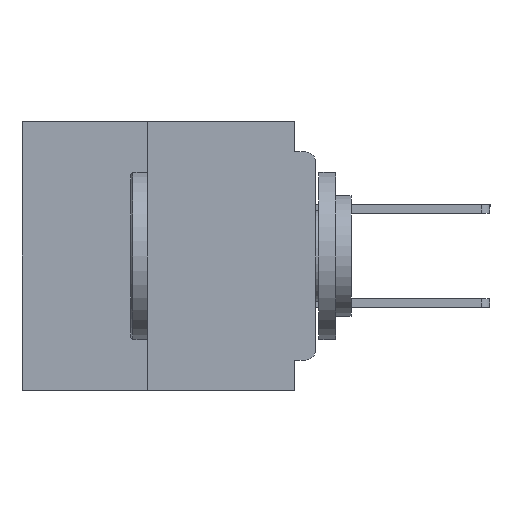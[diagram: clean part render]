
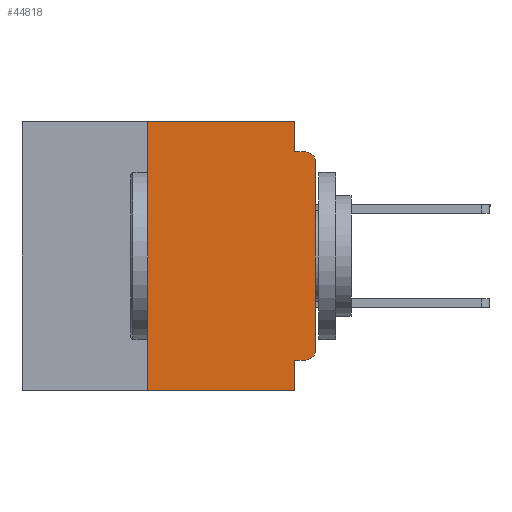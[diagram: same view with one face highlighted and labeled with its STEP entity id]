
A CAD part, left-side view. The second image highlights one B-rep face of the part: STEP entity #44818.
In plain terms, the highlighted planar face has unit normal (-1, 0, 0).
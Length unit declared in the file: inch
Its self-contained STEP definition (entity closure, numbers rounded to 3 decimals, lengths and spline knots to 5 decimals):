
#146 = EDGE_CURVE ( 'NONE', #15753, #48713, #27996, .T. ) ;
#553 = CARTESIAN_POINT ( 'NONE',  ( 0., 0.031, -0.4 ) ) ;
#1246 = AXIS2_PLACEMENT_3D ( 'NONE', #45370, #20375, #49547 ) ;
#2665 = EDGE_CURVE ( 'NONE', #50250, #47781, #18035, .T. ) ;
#3041 = CARTESIAN_POINT ( 'NONE',  ( 0., 0.25, 0. ) ) ;
#3782 = ORIENTED_EDGE ( 'NONE', *, *, #18799, .F. ) ;
#4461 = ORIENTED_EDGE ( 'NONE', *, *, #39982, .F. ) ;
#4476 = CARTESIAN_POINT ( 'NONE',  ( 0., 0.031, 0. ) ) ;
#5302 = DIRECTION ( 'NONE',  ( -1., 0., 0. ) ) ;
#5650 = VECTOR ( 'NONE', #20246, 39.37008 ) ;
#5683 = VERTEX_POINT ( 'NONE', #52691 ) ;
#5891 = ORIENTED_EDGE ( 'NONE', *, *, #11629, .F. ) ;
#6743 = LINE ( 'NONE', #34945, #38711 ) ;
#7755 = CIRCLE ( 'NONE', #17755, 0.015 ) ;
#7781 = CARTESIAN_POINT ( 'NONE',  ( 0., 0.437, -0.4 ) ) ;
#8504 = CARTESIAN_POINT ( 'NONE',  ( 0., 0.25, -0.4 ) ) ;
#9995 = DIRECTION ( 'NONE',  ( 0., 0., -1. ) ) ;
#11583 = CARTESIAN_POINT ( 'NONE',  ( 0., 0., -0.355 ) ) ;
#11629 = EDGE_CURVE ( 'NONE', #36801, #22110, #16083, .T. ) ;
#14085 = ORIENTED_EDGE ( 'NONE', *, *, #23699, .T. ) ;
#14198 = CARTESIAN_POINT ( 'NONE',  ( 0., 0., -0.045 ) ) ;
#14238 = ORIENTED_EDGE ( 'NONE', *, *, #2665, .F. ) ;
#14779 = VECTOR ( 'NONE', #30778, 39.37008 ) ;
#15753 = VERTEX_POINT ( 'NONE', #40698 ) ;
#15773 = VECTOR ( 'NONE', #40777, 39.37008 ) ;
#16083 = LINE ( 'NONE', #14198, #14779 ) ;
#16989 = ORIENTED_EDGE ( 'NONE', *, *, #146, .T. ) ;
#17755 = AXIS2_PLACEMENT_3D ( 'NONE', #30253, #5302, #34448 ) ;
#17911 = ORIENTED_EDGE ( 'NONE', *, *, #20209, .T. ) ;
#18035 = LINE ( 'NONE', #32659, #5650 ) ;
#18799 = EDGE_CURVE ( 'NONE', #47781, #30385, #25521, .T. ) ;
#20010 = DIRECTION ( 'NONE',  ( 0., 0., -1. ) ) ;
#20209 = EDGE_CURVE ( 'NONE', #31880, #22110, #7755, .T. ) ;
#20246 = DIRECTION ( 'NONE',  ( 0., 0., 1. ) ) ;
#20375 = DIRECTION ( 'NONE',  ( 1., 0., 0. ) ) ;
#22110 = VERTEX_POINT ( 'NONE', #34805 ) ;
#22960 = LINE ( 'NONE', #41863, #53618 ) ;
#23041 = ORIENTED_EDGE ( 'NONE', *, *, #51863, .T. ) ;
#23189 = CARTESIAN_POINT ( 'NONE',  ( 0., 0.015, -0.34 ) ) ;
#23251 = DIRECTION ( 'NONE',  ( 0., 0., 1. ) ) ;
#23699 = EDGE_CURVE ( 'NONE', #50250, #24543, #30273, .T. ) ;
#24200 = EDGE_LOOP ( 'NONE', ( #23041, #17911, #5891, #34847, #3782, #14238, #14085, #4461, #45010, #16989 ) ) ;
#24543 = VERTEX_POINT ( 'NONE', #553 ) ;
#25521 = LINE ( 'NONE', #51788, #47712 ) ;
#25557 = LINE ( 'NONE', #11583, #15773 ) ;
#25591 = EDGE_CURVE ( 'NONE', #15753, #5683, #25557, .T. ) ;
#27295 = CARTESIAN_POINT ( 'NONE',  ( 0., 0., 0. ) ) ;
#27996 = CIRCLE ( 'NONE', #41090, 0.015 ) ;
#30253 = CARTESIAN_POINT ( 'NONE',  ( 0., 0.015, -0.06 ) ) ;
#30273 = LINE ( 'NONE', #7781, #52391 ) ;
#30385 = VERTEX_POINT ( 'NONE', #4476 ) ;
#30778 = DIRECTION ( 'NONE',  ( 0., -1., 0. ) ) ;
#31880 = VERTEX_POINT ( 'NONE', #40984 ) ;
#32659 = CARTESIAN_POINT ( 'NONE',  ( 0., 0.25, -0.4 ) ) ;
#33139 = VECTOR ( 'NONE', #23251, 39.37008 ) ;
#33639 = DIRECTION ( 'NONE',  ( 0., 0., -1. ) ) ;
#34111 = DIRECTION ( 'NONE',  ( -1., 0., 0. ) ) ;
#34448 = DIRECTION ( 'NONE',  ( 0., 0., -1. ) ) ;
#34805 = CARTESIAN_POINT ( 'NONE',  ( 0., 0.015, -0.045 ) ) ;
#34847 = ORIENTED_EDGE ( 'NONE', *, *, #36135, .F. ) ;
#34945 = CARTESIAN_POINT ( 'NONE',  ( 0., 0.031, 0. ) ) ;
#36135 = EDGE_CURVE ( 'NONE', #30385, #36801, #6743, .T. ) ;
#36801 = VERTEX_POINT ( 'NONE', #51798 ) ;
#37004 = PLANE ( 'NONE',  #1246 ) ;
#38711 = VECTOR ( 'NONE', #9995, 39.37008 ) ;
#39259 = DIRECTION ( 'NONE',  ( 0., -1., 0. ) ) ;
#39982 = EDGE_CURVE ( 'NONE', #5683, #24543, #22960, .T. ) ;
#40698 = CARTESIAN_POINT ( 'NONE',  ( 0., 0.015, -0.355 ) ) ;
#40777 = DIRECTION ( 'NONE',  ( 0., 1., 0. ) ) ;
#40984 = CARTESIAN_POINT ( 'NONE',  ( 0., 0., -0.06 ) ) ;
#41090 = AXIS2_PLACEMENT_3D ( 'NONE', #23189, #34111, #20010 ) ;
#41151 = DIRECTION ( 'NONE',  ( 0., -1., 0. ) ) ;
#41863 = CARTESIAN_POINT ( 'NONE',  ( 0., 0.031, -0.4 ) ) ;
#42337 = CARTESIAN_POINT ( 'NONE',  ( 0., 0., -0.34 ) ) ;
#44202 = LINE ( 'NONE', #27295, #33139 ) ;
#44818 = ADVANCED_FACE ( 'NONE', ( #49174 ), #37004, .F. ) ;
#45010 = ORIENTED_EDGE ( 'NONE', *, *, #25591, .F. ) ;
#45370 = CARTESIAN_POINT ( 'NONE',  ( 0., 0.437, 0. ) ) ;
#47712 = VECTOR ( 'NONE', #39259, 39.37008 ) ;
#47781 = VERTEX_POINT ( 'NONE', #3041 ) ;
#48713 = VERTEX_POINT ( 'NONE', #42337 ) ;
#49174 = FACE_OUTER_BOUND ( 'NONE', #24200, .T. ) ;
#49547 = DIRECTION ( 'NONE',  ( 0., 0., -1. ) ) ;
#50250 = VERTEX_POINT ( 'NONE', #8504 ) ;
#51788 = CARTESIAN_POINT ( 'NONE',  ( 0., 0.437, 0. ) ) ;
#51798 = CARTESIAN_POINT ( 'NONE',  ( 0., 0.031, -0.045 ) ) ;
#51863 = EDGE_CURVE ( 'NONE', #48713, #31880, #44202, .T. ) ;
#52391 = VECTOR ( 'NONE', #41151, 39.37008 ) ;
#52691 = CARTESIAN_POINT ( 'NONE',  ( 0., 0.031, -0.355 ) ) ;
#53618 = VECTOR ( 'NONE', #33639, 39.37008 ) ;
